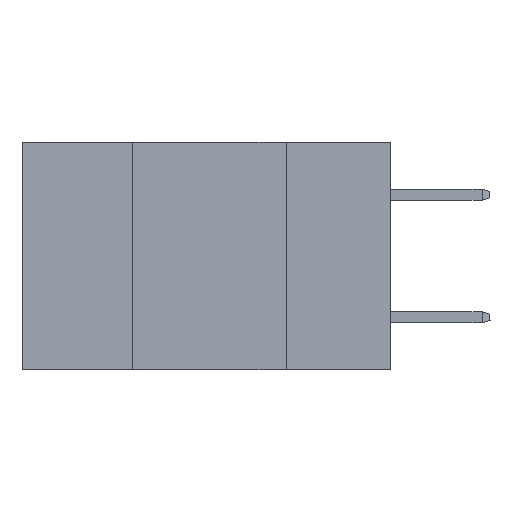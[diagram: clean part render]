
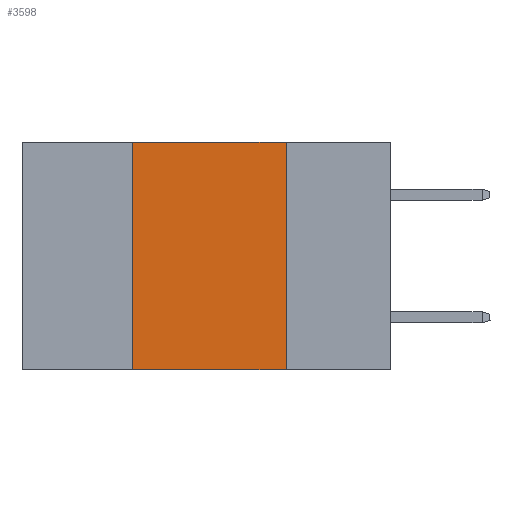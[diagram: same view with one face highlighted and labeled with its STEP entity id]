
A CAD part, left-side view. The second image highlights one B-rep face of the part: STEP entity #3598.
In plain terms, the highlighted planar face has unit normal (-1, 0, 0).
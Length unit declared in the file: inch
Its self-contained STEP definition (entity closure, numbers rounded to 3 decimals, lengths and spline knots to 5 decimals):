
#1990 = DIRECTION ( 'NONE',  ( 0., 0., 1. ) ) ;
#2326 = ORIENTED_EDGE ( 'NONE', *, *, #3149, .F. ) ;
#2751 = VECTOR ( 'NONE', #3398, 39.37008 ) ;
#2782 = VECTOR ( 'NONE', #8794, 39.37008 ) ;
#3149 = EDGE_CURVE ( 'NONE', #13974, #13576, #10776, .T. ) ;
#3264 = CARTESIAN_POINT ( 'NONE',  ( 0., 0.6, 0. ) ) ;
#3345 = CARTESIAN_POINT ( 'NONE',  ( 0., 0.6, 0. ) ) ;
#3398 = DIRECTION ( 'NONE',  ( 0., -1., 0. ) ) ;
#3598 = ADVANCED_FACE ( 'NONE', ( #13864 ), #5867, .F. ) ;
#4915 = DIRECTION ( 'NONE',  ( 1., 0., 0. ) ) ;
#4960 = DIRECTION ( 'NONE',  ( 0., 0., -1. ) ) ;
#5223 = LINE ( 'NONE', #13236, #8047 ) ;
#5648 = VERTEX_POINT ( 'NONE', #7463 ) ;
#5867 = PLANE ( 'NONE',  #13884 ) ;
#6286 = VERTEX_POINT ( 'NONE', #9119 ) ;
#6607 = CARTESIAN_POINT ( 'NONE',  ( 0., 0.42, 0. ) ) ;
#7052 = LINE ( 'NONE', #6607, #12412 ) ;
#7463 = CARTESIAN_POINT ( 'NONE',  ( 0., 0.17, -0.37 ) ) ;
#7544 = EDGE_CURVE ( 'NONE', #6286, #5648, #9019, .T. ) ;
#8047 = VECTOR ( 'NONE', #11212, 39.37008 ) ;
#8794 = DIRECTION ( 'NONE',  ( 0., -1., 0. ) ) ;
#8902 = ORIENTED_EDGE ( 'NONE', *, *, #7544, .T. ) ;
#9019 = LINE ( 'NONE', #13852, #2782 ) ;
#9119 = CARTESIAN_POINT ( 'NONE',  ( 0., 0.42, -0.37 ) ) ;
#9846 = EDGE_LOOP ( 'NONE', ( #11015, #2326, #13976, #8902 ) ) ;
#10776 = LINE ( 'NONE', #3264, #2751 ) ;
#11015 = ORIENTED_EDGE ( 'NONE', *, *, #11442, .F. ) ;
#11212 = DIRECTION ( 'NONE',  ( 0., 0., -1. ) ) ;
#11442 = EDGE_CURVE ( 'NONE', #13576, #5648, #5223, .T. ) ;
#12365 = CARTESIAN_POINT ( 'NONE',  ( 0., 0.42, 0. ) ) ;
#12412 = VECTOR ( 'NONE', #1990, 39.37008 ) ;
#13236 = CARTESIAN_POINT ( 'NONE',  ( 0., 0.17, 0. ) ) ;
#13576 = VERTEX_POINT ( 'NONE', #13862 ) ;
#13681 = EDGE_CURVE ( 'NONE', #6286, #13974, #7052, .T. ) ;
#13852 = CARTESIAN_POINT ( 'NONE',  ( 0., 0.6, -0.37 ) ) ;
#13862 = CARTESIAN_POINT ( 'NONE',  ( 0., 0.17, 0. ) ) ;
#13864 = FACE_OUTER_BOUND ( 'NONE', #9846, .T. ) ;
#13884 = AXIS2_PLACEMENT_3D ( 'NONE', #3345, #4915, #4960 ) ;
#13974 = VERTEX_POINT ( 'NONE', #12365 ) ;
#13976 = ORIENTED_EDGE ( 'NONE', *, *, #13681, .F. ) ;
